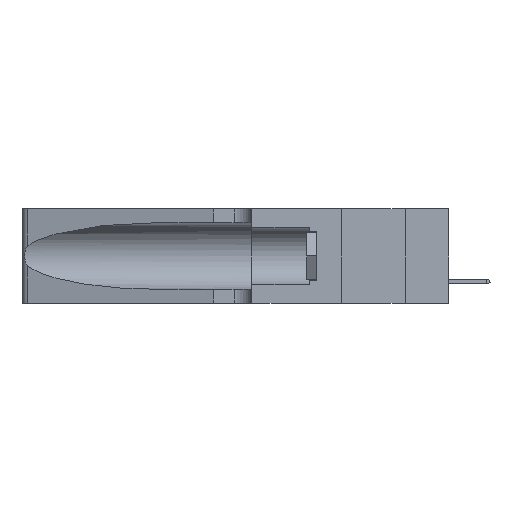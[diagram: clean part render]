
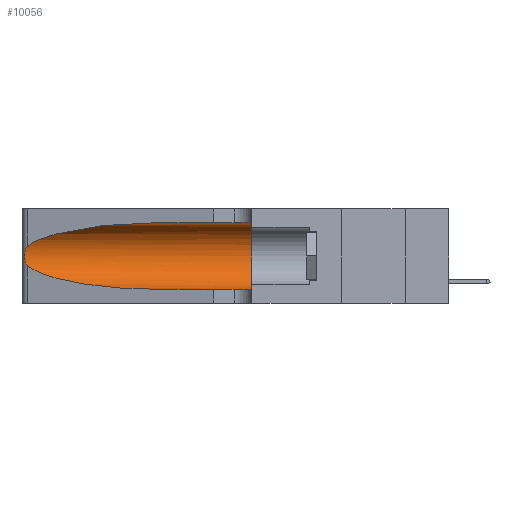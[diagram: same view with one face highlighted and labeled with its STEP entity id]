
A CAD part, left-side view. The second image highlights one B-rep face of the part: STEP entity #10056.
In plain terms, the highlighted cylindrical face has radius 3.308 mm (diameter 6.617 mm), a partial arc.
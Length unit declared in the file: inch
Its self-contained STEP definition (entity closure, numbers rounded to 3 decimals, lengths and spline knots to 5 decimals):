
#911 = FACE_OUTER_BOUND ( 'NONE', #16407, .T. ) ;
#1881 = LINE ( 'NONE', #8960, #11711 ) ;
#1944 = ORIENTED_EDGE ( 'NONE', *, *, #2718, .T. ) ;
#2527 =( BOUNDED_CURVE ( )  B_SPLINE_CURVE ( 3, ( #11227, #2752, #14220, #7014 ),
 .UNSPECIFIED., .F., .F. ) 
 B_SPLINE_CURVE_WITH_KNOTS ( ( 4, 4 ),
 ( 1.5708, 2.84003 ),
 .UNSPECIFIED. ) 
 CURVE ( )  GEOMETRIC_REPRESENTATION_ITEM ( )  RATIONAL_B_SPLINE_CURVE ( ( 1., 0.87, 0.87, 1. ) ) 
 REPRESENTATION_ITEM ( '' )  );
#2589 = ORIENTED_EDGE ( 'NONE', *, *, #15042, .T. ) ;
#2718 = EDGE_CURVE ( 'NONE', #5657, #7863, #1881, .T. ) ;
#2752 = CARTESIAN_POINT ( 'NONE',  ( 0.18966, 0.96281, 0.31525 ) ) ;
#3093 = CARTESIAN_POINT ( 'NONE',  ( 0.1305, 0.35, 0.185 ) ) ;
#3303 = CARTESIAN_POINT ( 'NONE',  ( 0.2373, 1.15595, 0.08982 ) ) ;
#3606 = VERTEX_POINT ( 'NONE', #14936 ) ;
#3793 = EDGE_CURVE ( 'NONE', #3606, #13366, #18168, .T. ) ;
#3977 = CARTESIAN_POINT ( 'NONE',  ( 0.25487, 1.22718, 0.14631 ) ) ;
#4365 = DIRECTION ( 'NONE',  ( 0., -1., 0. ) ) ;
#4514 = CYLINDRICAL_SURFACE ( 'NONE', #14280, 0.13025 ) ;
#4537 = DIRECTION ( 'NONE',  ( 0., 0., 1. ) ) ;
#4555 = CARTESIAN_POINT ( 'NONE',  ( 0.18966, 0.96281, 0.05475 ) ) ;
#4599 = EDGE_CURVE ( 'NONE', #13366, #7863, #15863, .T. ) ;
#5655 = CARTESIAN_POINT ( 'NONE',  ( 0.25639, 1.23186, 0.15144 ) ) ;
#5657 = VERTEX_POINT ( 'NONE', #8549 ) ;
#6170 = CARTESIAN_POINT ( 'NONE',  ( 0.25487, 1.22718, 0.14631 ) ) ;
#6894 = CARTESIAN_POINT ( 'NONE',  ( 0.1305, 0.35, 0.31525 ) ) ;
#7014 = CARTESIAN_POINT ( 'NONE',  ( 0.25487, 1.22718, 0.22369 ) ) ;
#7106 = CARTESIAN_POINT ( 'NONE',  ( 0.1305, 1.61858, 0.185 ) ) ;
#7165 = DIRECTION ( 'NONE',  ( 0., 0., -1. ) ) ;
#7287 = CARTESIAN_POINT ( 'NONE',  ( 0.26018, 1.23835, 0.19895 ) ) ;
#7570 = CARTESIAN_POINT ( 'NONE',  ( 0.25487, 1.22718, 0.22369 ) ) ;
#7863 = VERTEX_POINT ( 'NONE', #14946 ) ;
#8261 = AXIS2_PLACEMENT_3D ( 'NONE', #3093, #13047, #4537 ) ;
#8467 = CARTESIAN_POINT ( 'NONE',  ( 0.25487, 1.22718, 0.14631 ) ) ;
#8549 = CARTESIAN_POINT ( 'NONE',  ( 0.1305, 0.72297, 0.05475 ) ) ;
#8591 = CARTESIAN_POINT ( 'NONE',  ( 0.26075, 1.23896, 0.19203 ) ) ;
#8848 = CARTESIAN_POINT ( 'NONE',  ( 0.1305, 0.72297, 0.05475 ) ) ;
#8960 = CARTESIAN_POINT ( 'NONE',  ( 0.1305, 1.61858, 0.05475 ) ) ;
#9168 =( BOUNDED_CURVE ( )  B_SPLINE_CURVE ( 3, ( #6170, #3303, #4555, #8848 ),
 .UNSPECIFIED., .F., .F. ) 
 B_SPLINE_CURVE_WITH_KNOTS ( ( 4, 4 ),
 ( 3.44316, 4.71239 ),
 .UNSPECIFIED. ) 
 CURVE ( )  GEOMETRIC_REPRESENTATION_ITEM ( )  RATIONAL_B_SPLINE_CURVE ( ( 1., 0.87, 0.87, 1. ) ) 
 REPRESENTATION_ITEM ( '' )  );
#9494 = B_SPLINE_CURVE_WITH_KNOTS ( 'NONE', 3,
 ( #9891, #14377, #11445, #12808, #12863, #7287, #8591, #14184, #15684, #15551, #17252, #5655, #14311, #8467 ),
 .UNSPECIFIED., .F., .F.,
 ( 4, 2, 2, 2, 2, 2, 4 ),
 ( 0., 0.00027, 0.00053, 0.00107, 0.0016, 0.00187, 0.00214 ),
 .UNSPECIFIED. ) ;
#9808 = DIRECTION ( 'NONE',  ( 0., -1., 0. ) ) ;
#9891 = CARTESIAN_POINT ( 'NONE',  ( 0.25487, 1.22718, 0.22369 ) ) ;
#10056 = ADVANCED_FACE ( 'NONE', ( #911 ), #4514, .F. ) ;
#10204 = EDGE_CURVE ( 'NONE', #14994, #5657, #9168, .T. ) ;
#10905 = ORIENTED_EDGE ( 'NONE', *, *, #3793, .F. ) ;
#11227 = CARTESIAN_POINT ( 'NONE',  ( 0.1305, 0.72297, 0.31525 ) ) ;
#11445 = CARTESIAN_POINT ( 'NONE',  ( 0.25639, 1.23184, 0.21858 ) ) ;
#11711 = VECTOR ( 'NONE', #11810, 39.37008 ) ;
#11798 = VERTEX_POINT ( 'NONE', #7570 ) ;
#11810 = DIRECTION ( 'NONE',  ( 0., -1., 0. ) ) ;
#11893 = ORIENTED_EDGE ( 'NONE', *, *, #10204, .T. ) ;
#12808 = CARTESIAN_POINT ( 'NONE',  ( 0.25787, 1.23484, 0.2124 ) ) ;
#12863 = CARTESIAN_POINT ( 'NONE',  ( 0.25854, 1.2359, 0.20912 ) ) ;
#13047 = DIRECTION ( 'NONE',  ( 0., 1., 0. ) ) ;
#13288 = EDGE_CURVE ( 'NONE', #3606, #11798, #2527, .T. ) ;
#13366 = VERTEX_POINT ( 'NONE', #6894 ) ;
#14184 = CARTESIAN_POINT ( 'NONE',  ( 0.26075, 1.23896, 0.178 ) ) ;
#14220 = CARTESIAN_POINT ( 'NONE',  ( 0.2373, 1.15595, 0.28018 ) ) ;
#14280 = AXIS2_PLACEMENT_3D ( 'NONE', #7106, #4365, #7165 ) ;
#14307 = ORIENTED_EDGE ( 'NONE', *, *, #4599, .F. ) ;
#14311 = CARTESIAN_POINT ( 'NONE',  ( 0.25555, 1.22993, 0.14849 ) ) ;
#14377 = CARTESIAN_POINT ( 'NONE',  ( 0.25555, 1.22994, 0.2215 ) ) ;
#14583 = VECTOR ( 'NONE', #9808, 39.37008 ) ;
#14936 = CARTESIAN_POINT ( 'NONE',  ( 0.1305, 0.72297, 0.31525 ) ) ;
#14946 = CARTESIAN_POINT ( 'NONE',  ( 0.1305, 0.35, 0.05475 ) ) ;
#14994 = VERTEX_POINT ( 'NONE', #3977 ) ;
#15042 = EDGE_CURVE ( 'NONE', #11798, #14994, #9494, .T. ) ;
#15551 = CARTESIAN_POINT ( 'NONE',  ( 0.25856, 1.23593, 0.16098 ) ) ;
#15684 = CARTESIAN_POINT ( 'NONE',  ( 0.26017, 1.23833, 0.17102 ) ) ;
#15863 = CIRCLE ( 'NONE', #8261, 0.13025 ) ;
#16407 = EDGE_LOOP ( 'NONE', ( #16916, #2589, #11893, #1944, #14307, #10905 ) ) ;
#16916 = ORIENTED_EDGE ( 'NONE', *, *, #13288, .T. ) ;
#17252 = CARTESIAN_POINT ( 'NONE',  ( 0.25789, 1.23486, 0.15765 ) ) ;
#18168 = LINE ( 'NONE', #18378, #14583 ) ;
#18378 = CARTESIAN_POINT ( 'NONE',  ( 0.1305, 1.61858, 0.31525 ) ) ;
